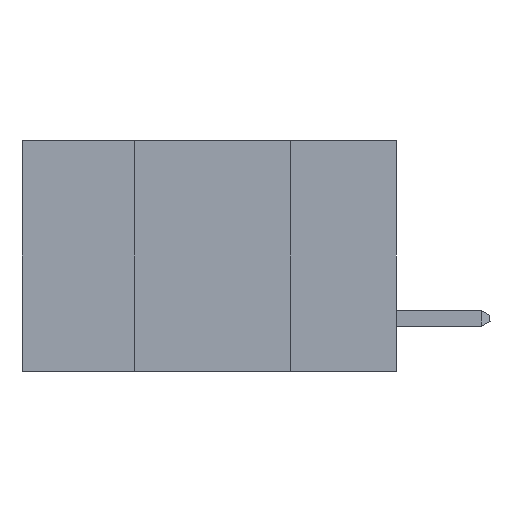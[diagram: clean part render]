
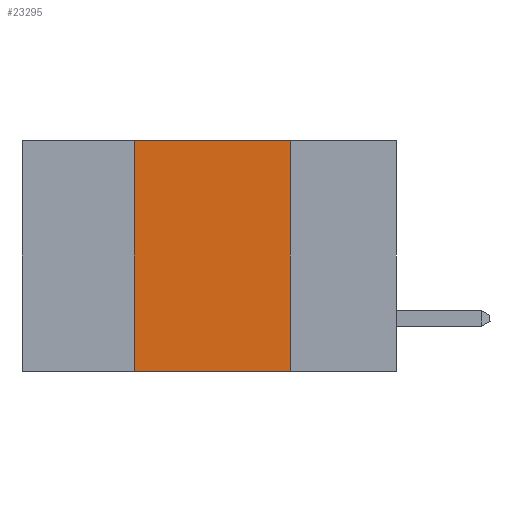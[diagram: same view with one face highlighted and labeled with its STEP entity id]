
A CAD part, left-side view. The second image highlights one B-rep face of the part: STEP entity #23295.
In plain terms, the highlighted planar face has unit normal (-1, 0, 0).
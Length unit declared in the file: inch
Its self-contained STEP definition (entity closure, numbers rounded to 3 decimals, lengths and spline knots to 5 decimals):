
#255 = EDGE_CURVE ( 'NONE', #4401, #12972, #346, .T. ) ;
#346 = LINE ( 'NONE', #9671, #18074 ) ;
#2044 = DIRECTION ( 'NONE',  ( 1., 0., 0. ) ) ;
#2143 = DIRECTION ( 'NONE',  ( 0., -1., 0. ) ) ;
#3357 = ORIENTED_EDGE ( 'NONE', *, *, #26081, .F. ) ;
#4053 = VERTEX_POINT ( 'NONE', #22726 ) ;
#4401 = VERTEX_POINT ( 'NONE', #16772 ) ;
#4513 = LINE ( 'NONE', #23143, #6831 ) ;
#5403 = VECTOR ( 'NONE', #20288, 39.37008 ) ;
#5532 = AXIS2_PLACEMENT_3D ( 'NONE', #12855, #2044, #6329 ) ;
#5744 = LINE ( 'NONE', #16404, #5403 ) ;
#6329 = DIRECTION ( 'NONE',  ( 0., 0., -1. ) ) ;
#6831 = VECTOR ( 'NONE', #16764, 39.37008 ) ;
#7020 = EDGE_CURVE ( 'NONE', #17088, #12972, #5744, .T. ) ;
#8166 = ORIENTED_EDGE ( 'NONE', *, *, #7020, .F. ) ;
#9562 = LINE ( 'NONE', #17389, #17569 ) ;
#9671 = CARTESIAN_POINT ( 'NONE',  ( 0., 0.6, -0.37 ) ) ;
#9841 = DIRECTION ( 'NONE',  ( 0., -1., 0. ) ) ;
#9884 = FACE_OUTER_BOUND ( 'NONE', #19001, .T. ) ;
#11516 = ORIENTED_EDGE ( 'NONE', *, *, #12788, .F. ) ;
#12174 = CARTESIAN_POINT ( 'NONE',  ( 0., 0.17, -0.37 ) ) ;
#12788 = EDGE_CURVE ( 'NONE', #4401, #4053, #4513, .T. ) ;
#12855 = CARTESIAN_POINT ( 'NONE',  ( 0., 0.6, 0. ) ) ;
#12972 = VERTEX_POINT ( 'NONE', #12174 ) ;
#16404 = CARTESIAN_POINT ( 'NONE',  ( 0., 0.17, 0. ) ) ;
#16764 = DIRECTION ( 'NONE',  ( 0., 0., 1. ) ) ;
#16772 = CARTESIAN_POINT ( 'NONE',  ( 0., 0.42, -0.37 ) ) ;
#17088 = VERTEX_POINT ( 'NONE', #24328 ) ;
#17389 = CARTESIAN_POINT ( 'NONE',  ( 0., 0.6, 0. ) ) ;
#17569 = VECTOR ( 'NONE', #2143, 39.37008 ) ;
#18074 = VECTOR ( 'NONE', #9841, 39.37008 ) ;
#18191 = ORIENTED_EDGE ( 'NONE', *, *, #255, .T. ) ;
#19001 = EDGE_LOOP ( 'NONE', ( #8166, #3357, #11516, #18191 ) ) ;
#19190 = PLANE ( 'NONE',  #5532 ) ;
#20288 = DIRECTION ( 'NONE',  ( 0., 0., -1. ) ) ;
#22726 = CARTESIAN_POINT ( 'NONE',  ( 0., 0.42, 0. ) ) ;
#23143 = CARTESIAN_POINT ( 'NONE',  ( 0., 0.42, 0. ) ) ;
#23295 = ADVANCED_FACE ( 'NONE', ( #9884 ), #19190, .F. ) ;
#24328 = CARTESIAN_POINT ( 'NONE',  ( 0., 0.17, 0. ) ) ;
#26081 = EDGE_CURVE ( 'NONE', #4053, #17088, #9562, .T. ) ;
